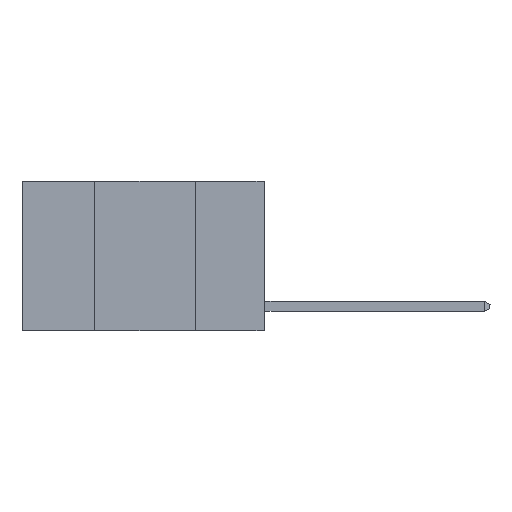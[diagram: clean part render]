
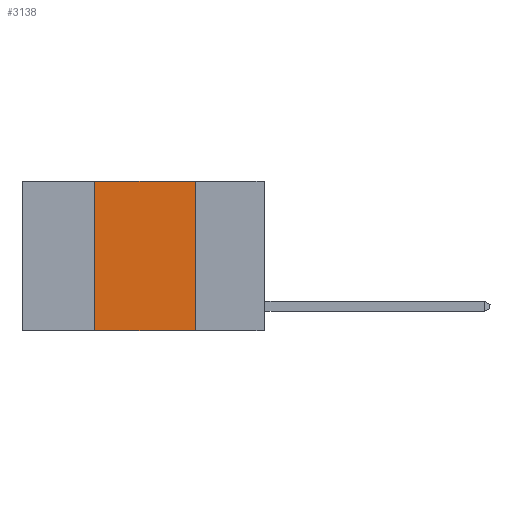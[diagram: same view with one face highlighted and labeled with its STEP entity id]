
A CAD part, left-side view. The second image highlights one B-rep face of the part: STEP entity #3138.
In plain terms, the highlighted planar face has unit normal (-1, 0, 0).
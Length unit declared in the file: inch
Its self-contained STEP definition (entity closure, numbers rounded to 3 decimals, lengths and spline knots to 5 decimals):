
#45 = DIRECTION ( 'NONE',  ( 0., 0., -1. ) ) ;
#126 = LINE ( 'NONE', #7156, #1146 ) ;
#466 = DIRECTION ( 'NONE',  ( 0., 0., 1. ) ) ;
#949 = ORIENTED_EDGE ( 'NONE', *, *, #3276, .F. ) ;
#1146 = VECTOR ( 'NONE', #12013, 39.37008 ) ;
#1185 = VECTOR ( 'NONE', #45, 39.37008 ) ;
#1432 = LINE ( 'NONE', #9390, #2176 ) ;
#1588 = EDGE_CURVE ( 'NONE', #11288, #4405, #9171, .T. ) ;
#1745 = AXIS2_PLACEMENT_3D ( 'NONE', #9957, #3114, #7224 ) ;
#2176 = VECTOR ( 'NONE', #466, 39.37008 ) ;
#3114 = DIRECTION ( 'NONE',  ( 1., 0., 0. ) ) ;
#3138 = ADVANCED_FACE ( 'NONE', ( #12730 ), #3955, .F. ) ;
#3276 = EDGE_CURVE ( 'NONE', #9116, #3938, #126, .T. ) ;
#3938 = VERTEX_POINT ( 'NONE', #4907 ) ;
#3955 = PLANE ( 'NONE',  #1745 ) ;
#4142 = ORIENTED_EDGE ( 'NONE', *, *, #4931, .F. ) ;
#4401 = EDGE_CURVE ( 'NONE', #11288, #9116, #1432, .T. ) ;
#4405 = VERTEX_POINT ( 'NONE', #5948 ) ;
#4625 = ORIENTED_EDGE ( 'NONE', *, *, #1588, .T. ) ;
#4824 = EDGE_LOOP ( 'NONE', ( #4142, #949, #10395, #4625 ) ) ;
#4907 = CARTESIAN_POINT ( 'NONE',  ( 0., 0.17, 0. ) ) ;
#4931 = EDGE_CURVE ( 'NONE', #3938, #4405, #8006, .T. ) ;
#5187 = CARTESIAN_POINT ( 'NONE',  ( 0., 0.6, -0.37 ) ) ;
#5839 = VECTOR ( 'NONE', #7285, 39.37008 ) ;
#5948 = CARTESIAN_POINT ( 'NONE',  ( 0., 0.17, -0.37 ) ) ;
#6004 = CARTESIAN_POINT ( 'NONE',  ( 0., 0.17, 0. ) ) ;
#7156 = CARTESIAN_POINT ( 'NONE',  ( 0., 0.6, 0. ) ) ;
#7224 = DIRECTION ( 'NONE',  ( 0., 0., -1. ) ) ;
#7285 = DIRECTION ( 'NONE',  ( 0., -1., 0. ) ) ;
#8006 = LINE ( 'NONE', #6004, #1185 ) ;
#9069 = CARTESIAN_POINT ( 'NONE',  ( 0., 0.42, -0.37 ) ) ;
#9116 = VERTEX_POINT ( 'NONE', #9381 ) ;
#9171 = LINE ( 'NONE', #5187, #5839 ) ;
#9381 = CARTESIAN_POINT ( 'NONE',  ( 0., 0.42, 0. ) ) ;
#9390 = CARTESIAN_POINT ( 'NONE',  ( 0., 0.42, 0. ) ) ;
#9957 = CARTESIAN_POINT ( 'NONE',  ( 0., 0.6, 0. ) ) ;
#10395 = ORIENTED_EDGE ( 'NONE', *, *, #4401, .F. ) ;
#11288 = VERTEX_POINT ( 'NONE', #9069 ) ;
#12013 = DIRECTION ( 'NONE',  ( 0., -1., 0. ) ) ;
#12730 = FACE_OUTER_BOUND ( 'NONE', #4824, .T. ) ;
